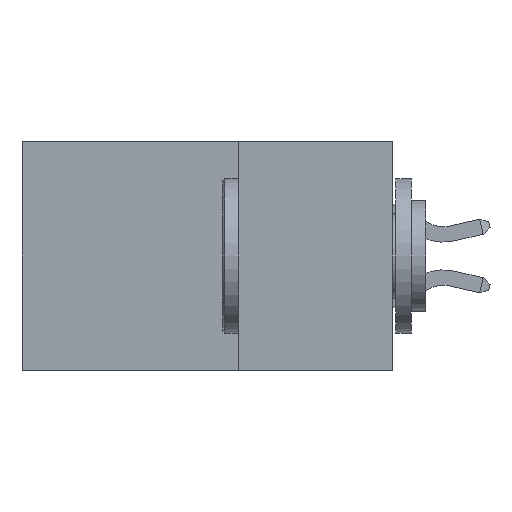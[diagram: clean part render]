
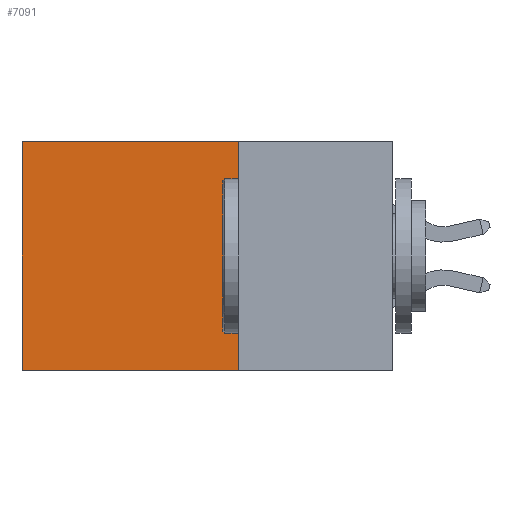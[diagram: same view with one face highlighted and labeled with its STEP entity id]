
A CAD part, left-side view. The second image highlights one B-rep face of the part: STEP entity #7091.
In plain terms, the highlighted planar face has unit normal (-1, 0, 0).
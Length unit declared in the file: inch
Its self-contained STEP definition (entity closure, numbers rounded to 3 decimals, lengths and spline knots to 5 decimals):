
#305 = ORIENTED_EDGE ( 'NONE', *, *, #9519, .F. ) ;
#595 = ORIENTED_EDGE ( 'NONE', *, *, #10438, .T. ) ;
#928 = FACE_OUTER_BOUND ( 'NONE', #5594, .T. ) ;
#1291 = LINE ( 'NONE', #4481, #10932 ) ;
#1686 = EDGE_CURVE ( 'NONE', #15143, #8102, #6843, .T. ) ;
#2804 = DIRECTION ( 'NONE',  ( 0., 1., 0. ) ) ;
#2869 = DIRECTION ( 'NONE',  ( 0., 0., -1. ) ) ;
#4352 = DIRECTION ( 'NONE',  ( 0., 0., -1. ) ) ;
#4358 = DIRECTION ( 'NONE',  ( 0., 0., -1. ) ) ;
#4481 = CARTESIAN_POINT ( 'NONE',  ( 0.2875, 0.25, 0. ) ) ;
#4484 = CARTESIAN_POINT ( 'NONE',  ( 0.2875, 0.6, 0. ) ) ;
#4892 = VERTEX_POINT ( 'NONE', #7737 ) ;
#5396 = ORIENTED_EDGE ( 'NONE', *, *, #18377, .T. ) ;
#5594 = EDGE_LOOP ( 'NONE', ( #5396, #10927, #305, #595 ) ) ;
#6843 = LINE ( 'NONE', #15521, #15081 ) ;
#7091 = ADVANCED_FACE ( 'NONE', ( #928 ), #8820, .F. ) ;
#7414 = VECTOR ( 'NONE', #4358, 39.37008 ) ;
#7737 = CARTESIAN_POINT ( 'NONE',  ( 0.2875, 0.6, 0. ) ) ;
#8102 = VERTEX_POINT ( 'NONE', #10802 ) ;
#8508 = LINE ( 'NONE', #11657, #13904 ) ;
#8820 = PLANE ( 'NONE',  #9097 ) ;
#9097 = AXIS2_PLACEMENT_3D ( 'NONE', #19382, #10352, #2869 ) ;
#9519 = EDGE_CURVE ( 'NONE', #16220, #15143, #1291, .T. ) ;
#9984 = DIRECTION ( 'NONE',  ( 0., 1., 0. ) ) ;
#10123 = CARTESIAN_POINT ( 'NONE',  ( 0.2875, 0.25, 0. ) ) ;
#10352 = DIRECTION ( 'NONE',  ( 1., 0., 0. ) ) ;
#10438 = EDGE_CURVE ( 'NONE', #16220, #4892, #8508, .T. ) ;
#10802 = CARTESIAN_POINT ( 'NONE',  ( 0.2875, 0.6, -0.37 ) ) ;
#10927 = ORIENTED_EDGE ( 'NONE', *, *, #1686, .F. ) ;
#10932 = VECTOR ( 'NONE', #4352, 39.37008 ) ;
#11657 = CARTESIAN_POINT ( 'NONE',  ( 0.2875, 0.25, 0. ) ) ;
#13904 = VECTOR ( 'NONE', #2804, 39.37008 ) ;
#15081 = VECTOR ( 'NONE', #9984, 39.37008 ) ;
#15143 = VERTEX_POINT ( 'NONE', #15990 ) ;
#15521 = CARTESIAN_POINT ( 'NONE',  ( 0.2875, 0.25, -0.37 ) ) ;
#15990 = CARTESIAN_POINT ( 'NONE',  ( 0.2875, 0.25, -0.37 ) ) ;
#16220 = VERTEX_POINT ( 'NONE', #10123 ) ;
#18377 = EDGE_CURVE ( 'NONE', #4892, #8102, #19468, .T. ) ;
#19382 = CARTESIAN_POINT ( 'NONE',  ( 0.2875, 0.25, 0. ) ) ;
#19468 = LINE ( 'NONE', #4484, #7414 ) ;
